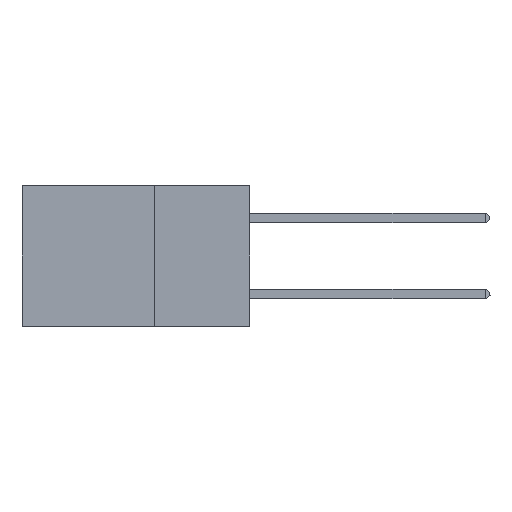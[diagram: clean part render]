
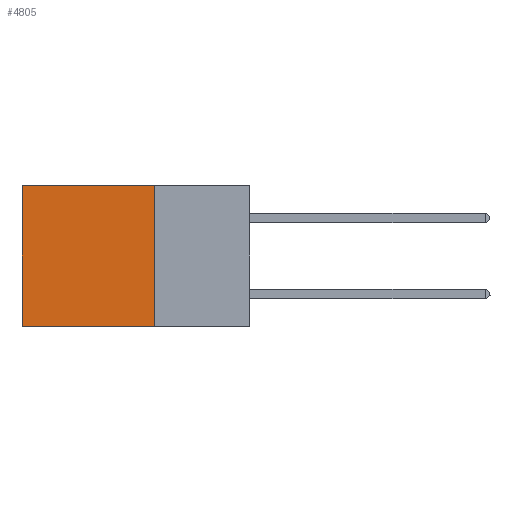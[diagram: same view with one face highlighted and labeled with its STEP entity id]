
A CAD part, left-side view. The second image highlights one B-rep face of the part: STEP entity #4805.
In plain terms, the highlighted planar face has unit normal (-1, 0, 0).
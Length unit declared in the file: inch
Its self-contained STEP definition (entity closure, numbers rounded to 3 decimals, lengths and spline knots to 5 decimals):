
#281 = VERTEX_POINT ( 'NONE', #9031 ) ;
#285 = ORIENTED_EDGE ( 'NONE', *, *, #3009, .T. ) ;
#681 = LINE ( 'NONE', #7053, #10316 ) ;
#785 = DIRECTION ( 'NONE',  ( 1., 0., 0. ) ) ;
#3009 = EDGE_CURVE ( 'NONE', #14418, #281, #7311, .T. ) ;
#3547 = CARTESIAN_POINT ( 'NONE',  ( 0.2875, 0.25, 0. ) ) ;
#3687 = ORIENTED_EDGE ( 'NONE', *, *, #6173, .F. ) ;
#4380 = DIRECTION ( 'NONE',  ( 0., 0., -1. ) ) ;
#4805 = ADVANCED_FACE ( 'NONE', ( #13847 ), #11083, .F. ) ;
#5164 = VECTOR ( 'NONE', #7913, 39.37008 ) ;
#5231 = VERTEX_POINT ( 'NONE', #10782 ) ;
#5255 = CARTESIAN_POINT ( 'NONE',  ( 0.2875, 0.25, -0.37 ) ) ;
#5851 = EDGE_CURVE ( 'NONE', #9294, #14418, #10447, .T. ) ;
#5870 = EDGE_CURVE ( 'NONE', #9294, #5231, #681, .T. ) ;
#6173 = EDGE_CURVE ( 'NONE', #5231, #281, #7778, .T. ) ;
#6504 = VECTOR ( 'NONE', #9785, 39.37008 ) ;
#7053 = CARTESIAN_POINT ( 'NONE',  ( 0.2875, 0.25, 0. ) ) ;
#7129 = ORIENTED_EDGE ( 'NONE', *, *, #5870, .F. ) ;
#7311 = LINE ( 'NONE', #13377, #5164 ) ;
#7778 = LINE ( 'NONE', #5255, #6504 ) ;
#7913 = DIRECTION ( 'NONE',  ( 0., 0., -1. ) ) ;
#8204 = DIRECTION ( 'NONE',  ( 0., 0., -1. ) ) ;
#9031 = CARTESIAN_POINT ( 'NONE',  ( 0.2875, 0.6, -0.37 ) ) ;
#9050 = EDGE_LOOP ( 'NONE', ( #285, #3687, #7129, #9843 ) ) ;
#9294 = VERTEX_POINT ( 'NONE', #3547 ) ;
#9785 = DIRECTION ( 'NONE',  ( 0., 1., 0. ) ) ;
#9843 = ORIENTED_EDGE ( 'NONE', *, *, #5851, .T. ) ;
#10101 = VECTOR ( 'NONE', #11704, 39.37008 ) ;
#10316 = VECTOR ( 'NONE', #8204, 39.37008 ) ;
#10447 = LINE ( 'NONE', #10477, #10101 ) ;
#10477 = CARTESIAN_POINT ( 'NONE',  ( 0.2875, 0.25, 0. ) ) ;
#10601 = AXIS2_PLACEMENT_3D ( 'NONE', #12277, #785, #4380 ) ;
#10782 = CARTESIAN_POINT ( 'NONE',  ( 0.2875, 0.25, -0.37 ) ) ;
#11083 = PLANE ( 'NONE',  #10601 ) ;
#11704 = DIRECTION ( 'NONE',  ( 0., 1., 0. ) ) ;
#12277 = CARTESIAN_POINT ( 'NONE',  ( 0.2875, 0.25, 0. ) ) ;
#13377 = CARTESIAN_POINT ( 'NONE',  ( 0.2875, 0.6, 0. ) ) ;
#13847 = FACE_OUTER_BOUND ( 'NONE', #9050, .T. ) ;
#14194 = CARTESIAN_POINT ( 'NONE',  ( 0.2875, 0.6, 0. ) ) ;
#14418 = VERTEX_POINT ( 'NONE', #14194 ) ;
